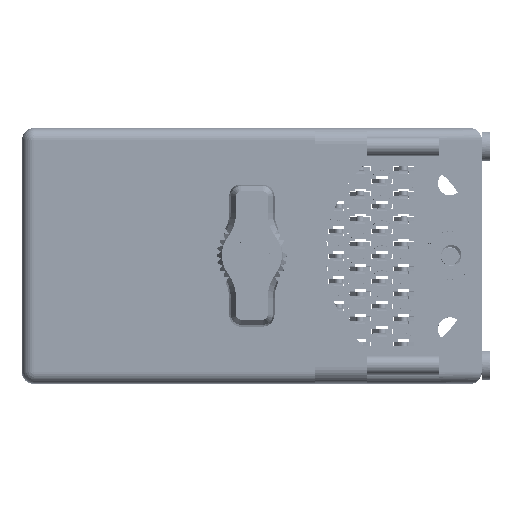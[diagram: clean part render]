
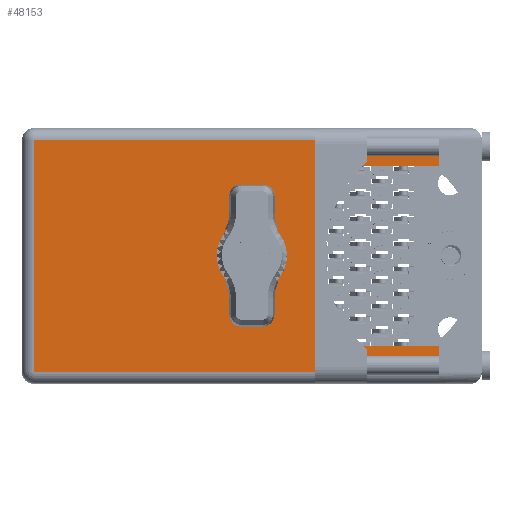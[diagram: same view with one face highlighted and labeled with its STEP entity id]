
A CAD part, top view. The second image highlights one B-rep face of the part: STEP entity #48153.
In plain terms, the highlighted face is planar.
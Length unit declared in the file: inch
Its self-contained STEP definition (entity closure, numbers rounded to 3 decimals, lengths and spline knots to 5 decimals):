
#2648 = LINE ( 'NONE', #102104, #57206 ) ;
#3218 = DIRECTION ( 'NONE',  ( 0., 0., 1. ) ) ;
#3559 = VECTOR ( 'NONE', #98061, 39.37008 ) ;
#3988 = CARTESIAN_POINT ( 'NONE',  ( 1.1215, 1.93, -0.765 ) ) ;
#4286 = CARTESIAN_POINT ( 'NONE',  ( 1.1215, 1.93, 0.695 ) ) ;
#8159 = CARTESIAN_POINT ( 'NONE',  ( 0.4075, 1.93, 0.54 ) ) ;
#9496 = CARTESIAN_POINT ( 'NONE',  ( 0.4075, 1.93, -0.54 ) ) ;
#10673 = VERTEX_POINT ( 'NONE', #106470 ) ;
#10977 = CARTESIAN_POINT ( 'NONE',  ( -1.3075, 1.93, 0.695 ) ) ;
#13666 = DIRECTION ( 'NONE',  ( 1., 0., 0. ) ) ;
#14164 = VECTOR ( 'NONE', #26003, 39.37008 ) ;
#17411 = CARTESIAN_POINT ( 'NONE',  ( 1.1215, 1.93, -0.54 ) ) ;
#17809 = CIRCLE ( 'NONE', #100445, 0.17 ) ;
#20023 = VERTEX_POINT ( 'NONE', #75754 ) ;
#22675 = EDGE_CURVE ( 'NONE', #10673, #87354, #2648, .T. ) ;
#22788 = DIRECTION ( 'NONE',  ( 0., 1., 0. ) ) ;
#24183 = DIRECTION ( 'NONE',  ( 0., 0., 1. ) ) ;
#24311 = CARTESIAN_POINT ( 'NONE',  ( -1.3775, 1.93, -0.765 ) ) ;
#24384 = EDGE_LOOP ( 'NONE', ( #92146, #44210, #62999, #60326, #90100, #55416, #38859, #70223 ) ) ;
#25608 = CARTESIAN_POINT ( 'NONE',  ( 0., 1.93, 0. ) ) ;
#26003 = DIRECTION ( 'NONE',  ( 1., 0., 0. ) ) ;
#26461 = CARTESIAN_POINT ( 'NONE',  ( 0.4075, 1.93, -0.54 ) ) ;
#32734 = CARTESIAN_POINT ( 'NONE',  ( 1.1215, 1.93, 0.54 ) ) ;
#33535 = VERTEX_POINT ( 'NONE', #32734 ) ;
#38858 = DIRECTION ( 'NONE',  ( 0., 0., 1. ) ) ;
#38859 = ORIENTED_EDGE ( 'NONE', *, *, #109266, .F. ) ;
#39025 = EDGE_CURVE ( 'NONE', #108022, #20023, #59022, .T. ) ;
#41371 = EDGE_LOOP ( 'NONE', ( #71016, #74497 ) ) ;
#44210 = ORIENTED_EDGE ( 'NONE', *, *, #109169, .T. ) ;
#47930 = EDGE_CURVE ( 'NONE', #20023, #108022, #17809, .T. ) ;
#48153 = ADVANCED_FACE ( 'NONE', ( #89085, #49989 ), #52098, .T. ) ;
#49989 = FACE_BOUND ( 'NONE', #41371, .T. ) ;
#51365 = CARTESIAN_POINT ( 'NONE',  ( 1.1215, 1.93, -0.54 ) ) ;
#52098 = PLANE ( 'NONE',  #62249 ) ;
#53871 = CARTESIAN_POINT ( 'NONE',  ( 1.1215, 1.93, 0.54 ) ) ;
#55416 = ORIENTED_EDGE ( 'NONE', *, *, #70408, .T. ) ;
#55428 = LINE ( 'NONE', #68433, #86172 ) ;
#56760 = LINE ( 'NONE', #87897, #63715 ) ;
#57206 = VECTOR ( 'NONE', #103284, 39.37008 ) ;
#57321 = LINE ( 'NONE', #3988, #114550 ) ;
#58967 = EDGE_CURVE ( 'NONE', #69729, #75373, #83355, .T. ) ;
#59022 = CIRCLE ( 'NONE', #109621, 0.17 ) ;
#60326 = ORIENTED_EDGE ( 'NONE', *, *, #112305, .T. ) ;
#61608 = DIRECTION ( 'NONE',  ( 0., 0., 1. ) ) ;
#62249 = AXIS2_PLACEMENT_3D ( 'NONE', #24311, #113782, #65921 ) ;
#62999 = ORIENTED_EDGE ( 'NONE', *, *, #106636, .F. ) ;
#63715 = VECTOR ( 'NONE', #24183, 39.37008 ) ;
#65921 = DIRECTION ( 'NONE',  ( -1., 0., 0. ) ) ;
#66613 = VERTEX_POINT ( 'NONE', #10977 ) ;
#66709 = VERTEX_POINT ( 'NONE', #4286 ) ;
#68433 = CARTESIAN_POINT ( 'NONE',  ( 1.1215, 1.93, 0.695 ) ) ;
#69729 = VERTEX_POINT ( 'NONE', #8159 ) ;
#70223 = ORIENTED_EDGE ( 'NONE', *, *, #22675, .T. ) ;
#70408 = EDGE_CURVE ( 'NONE', #75373, #114687, #82699, .T. ) ;
#71016 = ORIENTED_EDGE ( 'NONE', *, *, #47930, .F. ) ;
#73841 = EDGE_CURVE ( 'NONE', #87354, #66613, #99075, .T. ) ;
#74497 = ORIENTED_EDGE ( 'NONE', *, *, #39025, .F. ) ;
#74545 = DIRECTION ( 'NONE',  ( -1., 0., 0. ) ) ;
#75373 = VERTEX_POINT ( 'NONE', #9496 ) ;
#75576 = CARTESIAN_POINT ( 'NONE',  ( -1.3075, 1.93, -0.765 ) ) ;
#75687 = VECTOR ( 'NONE', #74545, 39.37008 ) ;
#75754 = CARTESIAN_POINT ( 'NONE',  ( 0., 1.93, 0.17 ) ) ;
#82699 = LINE ( 'NONE', #17411, #14164 ) ;
#83355 = LINE ( 'NONE', #26461, #3559 ) ;
#85738 = DIRECTION ( 'NONE',  ( 0., 0., 1. ) ) ;
#86070 = CARTESIAN_POINT ( 'NONE',  ( -1.3075, 1.93, -0.695 ) ) ;
#86172 = VECTOR ( 'NONE', #13666, 39.37008 ) ;
#87354 = VERTEX_POINT ( 'NONE', #86070 ) ;
#87897 = CARTESIAN_POINT ( 'NONE',  ( 1.1215, 1.93, -0.765 ) ) ;
#88235 = LINE ( 'NONE', #53871, #75687 ) ;
#89085 = FACE_OUTER_BOUND ( 'NONE', #24384, .T. ) ;
#90100 = ORIENTED_EDGE ( 'NONE', *, *, #58967, .T. ) ;
#92146 = ORIENTED_EDGE ( 'NONE', *, *, #73841, .T. ) ;
#98061 = DIRECTION ( 'NONE',  ( 0., 0., -1. ) ) ;
#99075 = LINE ( 'NONE', #75576, #105977 ) ;
#100445 = AXIS2_PLACEMENT_3D ( 'NONE', #102931, #22788, #85738 ) ;
#102104 = CARTESIAN_POINT ( 'NONE',  ( -1.3775, 1.93, -0.695 ) ) ;
#102931 = CARTESIAN_POINT ( 'NONE',  ( 0., 1.93, 0. ) ) ;
#103284 = DIRECTION ( 'NONE',  ( -1., 0., 0. ) ) ;
#105977 = VECTOR ( 'NONE', #38858, 39.37008 ) ;
#106470 = CARTESIAN_POINT ( 'NONE',  ( 1.1215, 1.93, -0.695 ) ) ;
#106636 = EDGE_CURVE ( 'NONE', #33535, #66709, #57321, .T. ) ;
#108022 = VERTEX_POINT ( 'NONE', #113129 ) ;
#109169 = EDGE_CURVE ( 'NONE', #66613, #66709, #55428, .T. ) ;
#109266 = EDGE_CURVE ( 'NONE', #10673, #114687, #56760, .T. ) ;
#109621 = AXIS2_PLACEMENT_3D ( 'NONE', #25608, #115048, #61608 ) ;
#112305 = EDGE_CURVE ( 'NONE', #33535, #69729, #88235, .T. ) ;
#113129 = CARTESIAN_POINT ( 'NONE',  ( 0., 1.93, -0.17 ) ) ;
#113782 = DIRECTION ( 'NONE',  ( 0., 1., 0. ) ) ;
#114550 = VECTOR ( 'NONE', #3218, 39.37008 ) ;
#114687 = VERTEX_POINT ( 'NONE', #51365 ) ;
#115048 = DIRECTION ( 'NONE',  ( 0., 1., 0. ) ) ;
